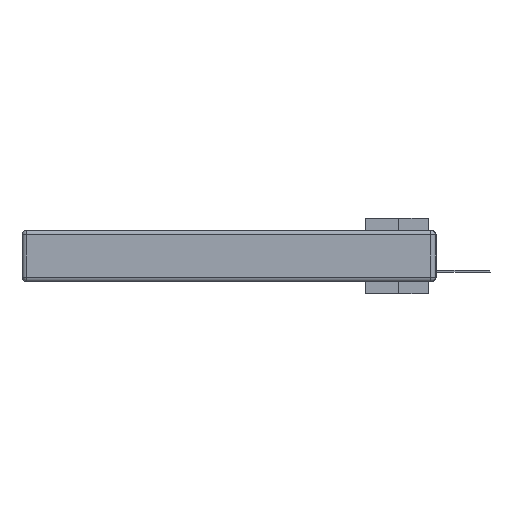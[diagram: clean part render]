
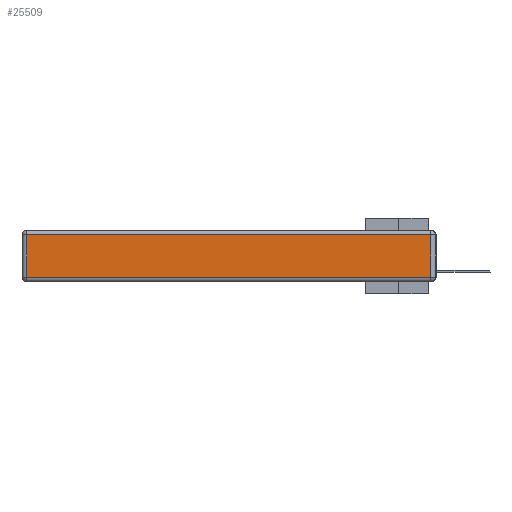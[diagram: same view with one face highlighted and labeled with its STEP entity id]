
A CAD part, left-side view. The second image highlights one B-rep face of the part: STEP entity #25509.
In plain terms, the highlighted planar face has unit normal (-1, 0, 0).
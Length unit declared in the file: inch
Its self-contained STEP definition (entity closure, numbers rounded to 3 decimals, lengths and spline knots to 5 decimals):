
#634 = LINE ( 'NONE', #11221, #3981 ) ;
#742 = VECTOR ( 'NONE', #5642, 39.37008 ) ;
#1175 = EDGE_CURVE ( 'NONE', #18101, #33641, #23125, .T. ) ;
#1522 = VECTOR ( 'NONE', #12115, 39.37008 ) ;
#3404 = CARTESIAN_POINT ( 'NONE',  ( 0., 0.03, -0.03 ) ) ;
#3507 = EDGE_LOOP ( 'NONE', ( #10853, #23896, #32838, #11569 ) ) ;
#3717 = CARTESIAN_POINT ( 'NONE',  ( 0., 0., -0.313 ) ) ;
#3981 = VECTOR ( 'NONE', #16556, 39.37008 ) ;
#5333 = VECTOR ( 'NONE', #6820, 39.37008 ) ;
#5642 = DIRECTION ( 'NONE',  ( 0., 0., -1. ) ) ;
#6786 = CARTESIAN_POINT ( 'NONE',  ( 0., 0.03, -0.313 ) ) ;
#6820 = DIRECTION ( 'NONE',  ( 0., -1., 0. ) ) ;
#6837 = DIRECTION ( 'NONE',  ( -1., 0., 0. ) ) ;
#8009 = EDGE_CURVE ( 'NONE', #16208, #14089, #634, .T. ) ;
#8913 = CARTESIAN_POINT ( 'NONE',  ( 0., 2.72, -0.03 ) ) ;
#9882 = PLANE ( 'NONE',  #14286 ) ;
#10853 = ORIENTED_EDGE ( 'NONE', *, *, #21719, .T. ) ;
#11221 = CARTESIAN_POINT ( 'NONE',  ( 0., 0.03, -0.343 ) ) ;
#11569 = ORIENTED_EDGE ( 'NONE', *, *, #1175, .T. ) ;
#12115 = DIRECTION ( 'NONE',  ( 0., 1., 0. ) ) ;
#12362 = EDGE_CURVE ( 'NONE', #14089, #18101, #20153, .T. ) ;
#14089 = VERTEX_POINT ( 'NONE', #3404 ) ;
#14286 = AXIS2_PLACEMENT_3D ( 'NONE', #15182, #6837, #30710 ) ;
#15182 = CARTESIAN_POINT ( 'NONE',  ( 0., 0., -0.343 ) ) ;
#16208 = VERTEX_POINT ( 'NONE', #6786 ) ;
#16556 = DIRECTION ( 'NONE',  ( 0., 0., 1. ) ) ;
#18101 = VERTEX_POINT ( 'NONE', #8913 ) ;
#20153 = LINE ( 'NONE', #32813, #1522 ) ;
#21490 = CARTESIAN_POINT ( 'NONE',  ( 0., 2.72, -0.343 ) ) ;
#21719 = EDGE_CURVE ( 'NONE', #33641, #16208, #33957, .T. ) ;
#23125 = LINE ( 'NONE', #21490, #742 ) ;
#23896 = ORIENTED_EDGE ( 'NONE', *, *, #8009, .T. ) ;
#25509 = ADVANCED_FACE ( 'NONE', ( #30857 ), #9882, .T. ) ;
#27639 = CARTESIAN_POINT ( 'NONE',  ( 0., 2.72, -0.313 ) ) ;
#30710 = DIRECTION ( 'NONE',  ( 0., 0., 1. ) ) ;
#30857 = FACE_OUTER_BOUND ( 'NONE', #3507, .T. ) ;
#32813 = CARTESIAN_POINT ( 'NONE',  ( 0., 2.75, -0.03 ) ) ;
#32838 = ORIENTED_EDGE ( 'NONE', *, *, #12362, .T. ) ;
#33641 = VERTEX_POINT ( 'NONE', #27639 ) ;
#33957 = LINE ( 'NONE', #3717, #5333 ) ;
